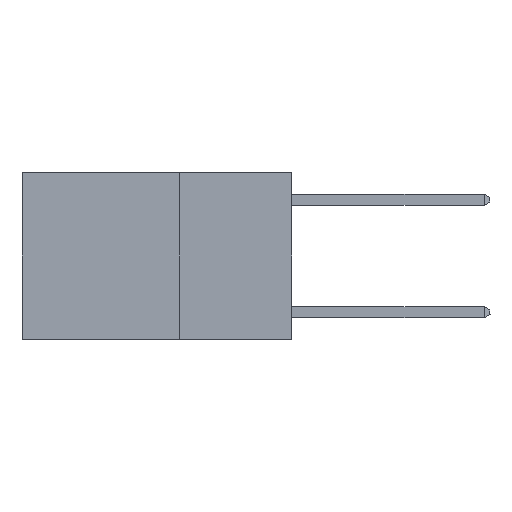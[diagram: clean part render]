
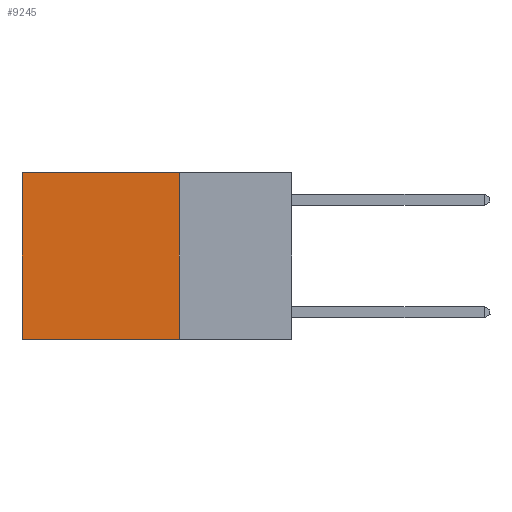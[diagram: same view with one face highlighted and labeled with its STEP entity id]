
A CAD part, left-side view. The second image highlights one B-rep face of the part: STEP entity #9245.
In plain terms, the highlighted planar face has unit normal (-1, 0, 0).
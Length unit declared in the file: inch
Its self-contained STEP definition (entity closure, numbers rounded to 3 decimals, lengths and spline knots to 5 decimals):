
#307 = VERTEX_POINT ( 'NONE', #10090 ) ;
#515 = EDGE_CURVE ( 'NONE', #307, #6995, #3925, .T. ) ;
#1007 = EDGE_CURVE ( 'NONE', #2108, #6995, #10703, .T. ) ;
#1032 = DIRECTION ( 'NONE',  ( 0., 0., -1. ) ) ;
#1483 = CARTESIAN_POINT ( 'NONE',  ( 0.2625, 0.25, 0. ) ) ;
#1635 = ORIENTED_EDGE ( 'NONE', *, *, #1007, .T. ) ;
#1942 = AXIS2_PLACEMENT_3D ( 'NONE', #10863, #6528, #1032 ) ;
#2108 = VERTEX_POINT ( 'NONE', #10231 ) ;
#2856 = CARTESIAN_POINT ( 'NONE',  ( 0.2625, 0.25, -0.37 ) ) ;
#3925 = LINE ( 'NONE', #2856, #10448 ) ;
#4091 = DIRECTION ( 'NONE',  ( 0., 1., 0. ) ) ;
#5165 = EDGE_CURVE ( 'NONE', #8903, #2108, #7083, .T. ) ;
#5516 = DIRECTION ( 'NONE',  ( 0., 0., -1. ) ) ;
#5589 = PLANE ( 'NONE',  #1942 ) ;
#5744 = VECTOR ( 'NONE', #10093, 39.37008 ) ;
#5801 = LINE ( 'NONE', #7303, #8189 ) ;
#6528 = DIRECTION ( 'NONE',  ( 1., 0., 0. ) ) ;
#6804 = VECTOR ( 'NONE', #11028, 39.37008 ) ;
#6884 = FACE_OUTER_BOUND ( 'NONE', #10273, .T. ) ;
#6995 = VERTEX_POINT ( 'NONE', #7028 ) ;
#7028 = CARTESIAN_POINT ( 'NONE',  ( 0.2625, 0.6, -0.37 ) ) ;
#7083 = LINE ( 'NONE', #10167, #6804 ) ;
#7190 = EDGE_CURVE ( 'NONE', #8903, #307, #5801, .T. ) ;
#7303 = CARTESIAN_POINT ( 'NONE',  ( 0.2625, 0.25, 0. ) ) ;
#7814 = CARTESIAN_POINT ( 'NONE',  ( 0.2625, 0.6, 0. ) ) ;
#8189 = VECTOR ( 'NONE', #5516, 39.37008 ) ;
#8549 = ORIENTED_EDGE ( 'NONE', *, *, #515, .F. ) ;
#8700 = ORIENTED_EDGE ( 'NONE', *, *, #7190, .F. ) ;
#8903 = VERTEX_POINT ( 'NONE', #1483 ) ;
#9245 = ADVANCED_FACE ( 'NONE', ( #6884 ), #5589, .F. ) ;
#9612 = ORIENTED_EDGE ( 'NONE', *, *, #5165, .T. ) ;
#10090 = CARTESIAN_POINT ( 'NONE',  ( 0.2625, 0.25, -0.37 ) ) ;
#10093 = DIRECTION ( 'NONE',  ( 0., 0., -1. ) ) ;
#10167 = CARTESIAN_POINT ( 'NONE',  ( 0.2625, 0.25, 0. ) ) ;
#10231 = CARTESIAN_POINT ( 'NONE',  ( 0.2625, 0.6, 0. ) ) ;
#10273 = EDGE_LOOP ( 'NONE', ( #1635, #8549, #8700, #9612 ) ) ;
#10448 = VECTOR ( 'NONE', #4091, 39.37008 ) ;
#10703 = LINE ( 'NONE', #7814, #5744 ) ;
#10863 = CARTESIAN_POINT ( 'NONE',  ( 0.2625, 0.25, 0. ) ) ;
#11028 = DIRECTION ( 'NONE',  ( 0., 1., 0. ) ) ;
